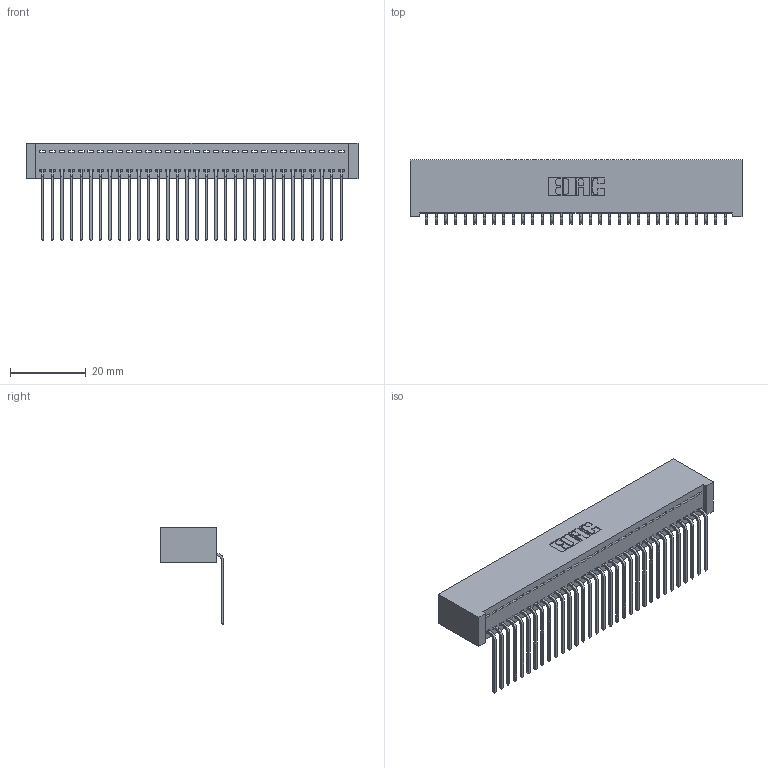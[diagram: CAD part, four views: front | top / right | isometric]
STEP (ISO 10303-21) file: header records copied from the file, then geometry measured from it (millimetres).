
FILE_DESCRIPTION (( 'STEP AP203' ), '1' );
FILE_NAME ('392-032-559-101.STEP', '2019-10-07T15:00:24', ( '' ), ( '' ), 'SwSTEP 2.0', 'SolidWorks 2016', '' );
FILE_SCHEMA (( 'CONFIG_CONTROL_DESIGN' ));
Length unit declared in the file: inch
Products named in the file (3): 342 Part_Lugless; 345-292-001_558 559 Tail - 1; 392-032-559-101
Assembly tree (33 placements, depth 2):
  392-032-559-101
    342 Part_Lugless
    345-292-001_558 559 Tail - 1  x32
Bounding box: 87.53 x 16.83 x 25.78 mm (x, y, z)
Volume: 8153.2 mm3; surface area: 12714.8 mm2
Topology: 33 solids, 33 shells, 2022 faces, 6099 edges, 4022 vertices
Faces by surface type: plane 1470, cylinder 552
Entity records: 20531 total; most frequent: CARTESIAN_POINT 3550, ORIENTED_EDGE 3518, DIRECTION 3007, EDGE_CURVE 1759, VECTOR 1639, LINE 1639, VERTEX_POINT 1170, AXIS2_PLACEMENT_3D 684
